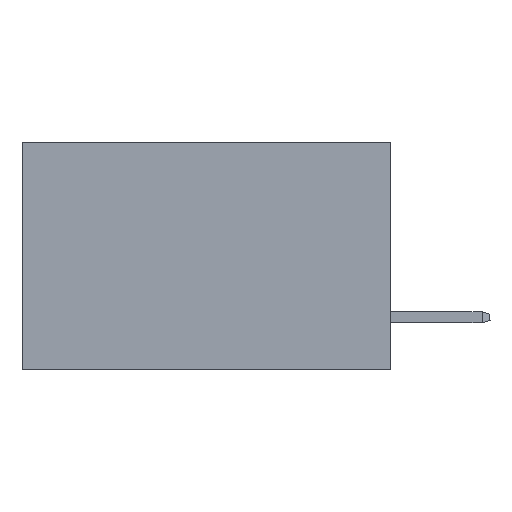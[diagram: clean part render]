
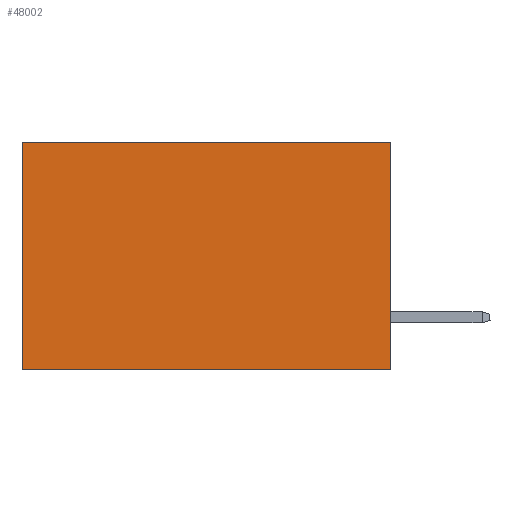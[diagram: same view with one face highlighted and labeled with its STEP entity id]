
A CAD part, left-side view. The second image highlights one B-rep face of the part: STEP entity #48002.
In plain terms, the highlighted planar face has unit normal (-1, 0, 0).
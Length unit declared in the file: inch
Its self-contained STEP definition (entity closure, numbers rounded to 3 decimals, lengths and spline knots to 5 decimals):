
#514 = VERTEX_POINT ( 'NONE', #6039 ) ;
#2840 = EDGE_CURVE ( 'NONE', #23029, #23457, #12287, .T. ) ;
#6039 = CARTESIAN_POINT ( 'NONE',  ( 0.2875, 0., -0.37 ) ) ;
#6254 = CARTESIAN_POINT ( 'NONE',  ( 0.2875, 0., 0. ) ) ;
#6928 = DIRECTION ( 'NONE',  ( 0., 0., -1. ) ) ;
#7373 = EDGE_CURVE ( 'NONE', #35089, #23029, #28752, .T. ) ;
#8685 = EDGE_CURVE ( 'NONE', #35089, #514, #43153, .T. ) ;
#10673 = VECTOR ( 'NONE', #17329, 39.37008 ) ;
#12287 = LINE ( 'NONE', #20071, #47843 ) ;
#13715 = ORIENTED_EDGE ( 'NONE', *, *, #7373, .T. ) ;
#14730 = CARTESIAN_POINT ( 'NONE',  ( 0.2875, 0.6, -0.37 ) ) ;
#14788 = VECTOR ( 'NONE', #36505, 39.37008 ) ;
#15748 = DIRECTION ( 'NONE',  ( 0., 0., -1. ) ) ;
#17329 = DIRECTION ( 'NONE',  ( 0., 1., 0. ) ) ;
#20071 = CARTESIAN_POINT ( 'NONE',  ( 0.2875, 0.6, 0. ) ) ;
#23029 = VERTEX_POINT ( 'NONE', #38183 ) ;
#23457 = VERTEX_POINT ( 'NONE', #14730 ) ;
#26221 = EDGE_LOOP ( 'NONE', ( #32822, #33155, #33262, #13715 ) ) ;
#28408 = CARTESIAN_POINT ( 'NONE',  ( 0.2875, 0., -0.37 ) ) ;
#28752 = LINE ( 'NONE', #39955, #14788 ) ;
#28788 = FACE_OUTER_BOUND ( 'NONE', #26221, .T. ) ;
#32188 = LINE ( 'NONE', #28408, #10673 ) ;
#32822 = ORIENTED_EDGE ( 'NONE', *, *, #2840, .T. ) ;
#33155 = ORIENTED_EDGE ( 'NONE', *, *, #38359, .F. ) ;
#33262 = ORIENTED_EDGE ( 'NONE', *, *, #8685, .F. ) ;
#34160 = DIRECTION ( 'NONE',  ( 1., 0., 0. ) ) ;
#34402 = AXIS2_PLACEMENT_3D ( 'NONE', #34484, #34160, #15748 ) ;
#34484 = CARTESIAN_POINT ( 'NONE',  ( 0.2875, 0., 0. ) ) ;
#35089 = VERTEX_POINT ( 'NONE', #6254 ) ;
#35117 = DIRECTION ( 'NONE',  ( 0., 0., -1. ) ) ;
#35596 = VECTOR ( 'NONE', #6928, 39.37008 ) ;
#35878 = CARTESIAN_POINT ( 'NONE',  ( 0.2875, 0., 0. ) ) ;
#36505 = DIRECTION ( 'NONE',  ( 0., 1., 0. ) ) ;
#38055 = PLANE ( 'NONE',  #34402 ) ;
#38183 = CARTESIAN_POINT ( 'NONE',  ( 0.2875, 0.6, 0. ) ) ;
#38359 = EDGE_CURVE ( 'NONE', #514, #23457, #32188, .T. ) ;
#39955 = CARTESIAN_POINT ( 'NONE',  ( 0.2875, 0., 0. ) ) ;
#43153 = LINE ( 'NONE', #35878, #35596 ) ;
#47843 = VECTOR ( 'NONE', #35117, 39.37008 ) ;
#48002 = ADVANCED_FACE ( 'NONE', ( #28788 ), #38055, .F. ) ;
